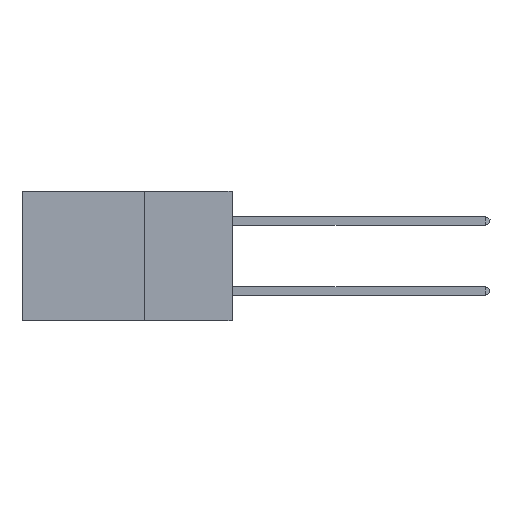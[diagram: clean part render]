
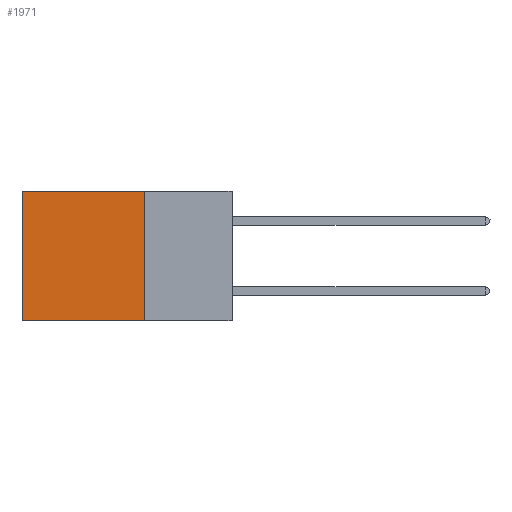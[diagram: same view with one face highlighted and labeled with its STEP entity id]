
A CAD part, left-side view. The second image highlights one B-rep face of the part: STEP entity #1971.
In plain terms, the highlighted planar face has unit normal (-1, 0, 0).
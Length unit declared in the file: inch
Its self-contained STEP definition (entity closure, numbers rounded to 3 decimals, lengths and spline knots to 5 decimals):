
#362 = AXIS2_PLACEMENT_3D ( 'NONE', #19956, #3040, #33255 ) ;
#673 = EDGE_CURVE ( 'NONE', #29004, #12308, #20699, .T. ) ;
#1971 = ADVANCED_FACE ( 'NONE', ( #8639 ), #26489, .F. ) ;
#2811 = CARTESIAN_POINT ( 'NONE',  ( 0.2875, 0.6, 0. ) ) ;
#3040 = DIRECTION ( 'NONE',  ( 1., 0., 0. ) ) ;
#3785 = VERTEX_POINT ( 'NONE', #2811 ) ;
#5387 = VECTOR ( 'NONE', #39562, 39.37008 ) ;
#6122 = CARTESIAN_POINT ( 'NONE',  ( 0.2875, 0.25, 0. ) ) ;
#7037 = DIRECTION ( 'NONE',  ( 0., 1., 0. ) ) ;
#8446 = EDGE_LOOP ( 'NONE', ( #14232, #23942, #31860, #38248 ) ) ;
#8639 = FACE_OUTER_BOUND ( 'NONE', #8446, .T. ) ;
#9359 = CARTESIAN_POINT ( 'NONE',  ( 0.2875, 0.25, 0. ) ) ;
#11450 = DIRECTION ( 'NONE',  ( 0., 0., -1. ) ) ;
#12308 = VERTEX_POINT ( 'NONE', #34936 ) ;
#14232 = ORIENTED_EDGE ( 'NONE', *, *, #41977, .T. ) ;
#15558 = CARTESIAN_POINT ( 'NONE',  ( 0.2875, 0.25, -0.37 ) ) ;
#16236 = VECTOR ( 'NONE', #35394, 39.37008 ) ;
#17669 = EDGE_CURVE ( 'NONE', #34370, #29004, #38402, .T. ) ;
#19838 = VECTOR ( 'NONE', #11450, 39.37008 ) ;
#19956 = CARTESIAN_POINT ( 'NONE',  ( 0.2875, 0.25, 0. ) ) ;
#20180 = EDGE_CURVE ( 'NONE', #34370, #3785, #21327, .T. ) ;
#20699 = LINE ( 'NONE', #15558, #28637 ) ;
#21327 = LINE ( 'NONE', #9359, #5387 ) ;
#23942 = ORIENTED_EDGE ( 'NONE', *, *, #673, .F. ) ;
#24161 = LINE ( 'NONE', #28737, #16236 ) ;
#25231 = CARTESIAN_POINT ( 'NONE',  ( 0.2875, 0.25, -0.37 ) ) ;
#26489 = PLANE ( 'NONE',  #362 ) ;
#28637 = VECTOR ( 'NONE', #7037, 39.37008 ) ;
#28737 = CARTESIAN_POINT ( 'NONE',  ( 0.2875, 0.6, 0. ) ) ;
#29004 = VERTEX_POINT ( 'NONE', #25231 ) ;
#31541 = CARTESIAN_POINT ( 'NONE',  ( 0.2875, 0.25, 0. ) ) ;
#31860 = ORIENTED_EDGE ( 'NONE', *, *, #17669, .F. ) ;
#33255 = DIRECTION ( 'NONE',  ( 0., 0., -1. ) ) ;
#34370 = VERTEX_POINT ( 'NONE', #6122 ) ;
#34936 = CARTESIAN_POINT ( 'NONE',  ( 0.2875, 0.6, -0.37 ) ) ;
#35394 = DIRECTION ( 'NONE',  ( 0., 0., -1. ) ) ;
#38248 = ORIENTED_EDGE ( 'NONE', *, *, #20180, .T. ) ;
#38402 = LINE ( 'NONE', #31541, #19838 ) ;
#39562 = DIRECTION ( 'NONE',  ( 0., 1., 0. ) ) ;
#41977 = EDGE_CURVE ( 'NONE', #3785, #12308, #24161, .T. ) ;
